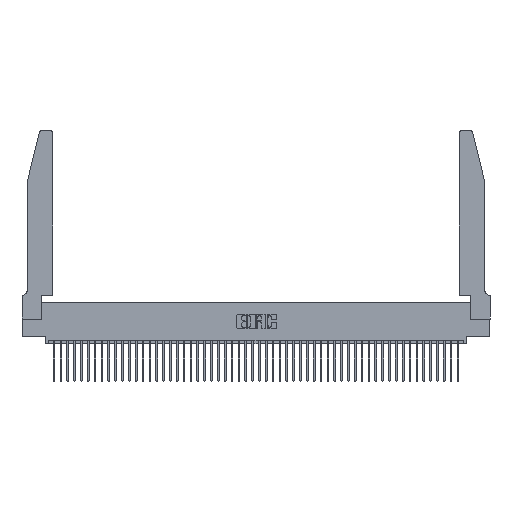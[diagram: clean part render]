
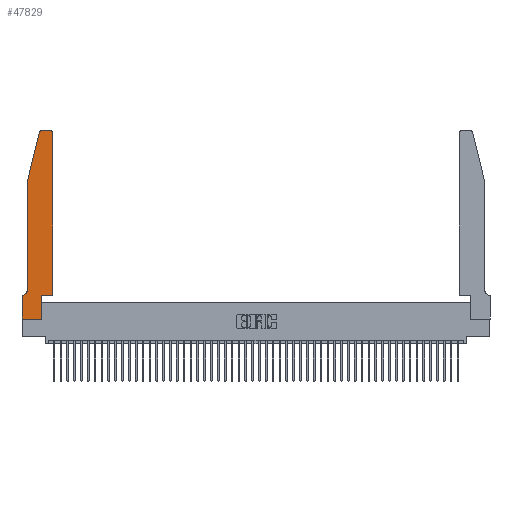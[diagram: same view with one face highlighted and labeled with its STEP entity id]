
A CAD part, top view. The second image highlights one B-rep face of the part: STEP entity #47829.
In plain terms, the highlighted planar face has unit normal (0, 0, 1).
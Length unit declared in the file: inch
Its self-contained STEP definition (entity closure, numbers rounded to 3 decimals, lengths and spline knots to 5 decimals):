
#329 = VERTEX_POINT ( 'NONE', #30062 ) ;
#383 = CARTESIAN_POINT ( 'NONE',  ( 0.2605, 2.75, 0.37 ) ) ;
#395 = LINE ( 'NONE', #383, #38813 ) ;
#433 = DIRECTION ( 'NONE',  ( 0., 0., 1. ) ) ;
#830 = EDGE_CURVE ( 'NONE', #15135, #20562, #17797, .T. ) ;
#2354 = LINE ( 'NONE', #9603, #21689 ) ;
#2930 = CARTESIAN_POINT ( 'NONE',  ( 0., 0., 0.37 ) ) ;
#4308 = DIRECTION ( 'NONE',  ( -1., 0., 0. ) ) ;
#4812 = DIRECTION ( 'NONE',  ( 1., 0., 0. ) ) ;
#5702 = FACE_OUTER_BOUND ( 'NONE', #33697, .T. ) ;
#6238 = CARTESIAN_POINT ( 'NONE',  ( 0.4205, 2.72, 0.37 ) ) ;
#7221 = VECTOR ( 'NONE', #25998, 39.37008 ) ;
#7371 = ORIENTED_EDGE ( 'NONE', *, *, #9291, .T. ) ;
#7664 = CARTESIAN_POINT ( 'NONE',  ( 0.0055, 0.42, 0.37 ) ) ;
#7694 = LINE ( 'NONE', #33181, #29290 ) ;
#8608 = EDGE_CURVE ( 'NONE', #26671, #40325, #7694, .T. ) ;
#9291 = EDGE_CURVE ( 'NONE', #26910, #37167, #21571, .T. ) ;
#9395 = AXIS2_PLACEMENT_3D ( 'NONE', #23550, #433, #27371 ) ;
#9603 = CARTESIAN_POINT ( 'NONE',  ( 0.0755, 2., 0.37 ) ) ;
#10123 = DIRECTION ( 'NONE',  ( 1., 0., 0. ) ) ;
#10576 = VECTOR ( 'NONE', #10858, 39.37008 ) ;
#10702 = CARTESIAN_POINT ( 'NONE',  ( 0.4205, 2.75, 0.37 ) ) ;
#10858 = DIRECTION ( 'NONE',  ( 0., -1., 0. ) ) ;
#11010 = VECTOR ( 'NONE', #29513, 39.37008 ) ;
#11382 = AXIS2_PLACEMENT_3D ( 'NONE', #7664, #34419, #11530 ) ;
#11530 = DIRECTION ( 'NONE',  ( -1., 0., 0. ) ) ;
#12657 = CARTESIAN_POINT ( 'NONE',  ( 0., 0.35, 0.37 ) ) ;
#12676 = CARTESIAN_POINT ( 'NONE',  ( 0.2865, 0.35, 0.37 ) ) ;
#13490 = DIRECTION ( 'NONE',  ( -0.239, -0.971, 0. ) ) ;
#13659 = DIRECTION ( 'NONE',  ( 0., -1., 0. ) ) ;
#14196 = ORIENTED_EDGE ( 'NONE', *, *, #830, .T. ) ;
#14727 = CARTESIAN_POINT ( 'NONE',  ( 0.0755, 0.42, 0.37 ) ) ;
#14884 = CIRCLE ( 'NONE', #9395, 0.03 ) ;
#15135 = VERTEX_POINT ( 'NONE', #15682 ) ;
#15682 = CARTESIAN_POINT ( 'NONE',  ( 0., 0.35, 0.37 ) ) ;
#16291 = CARTESIAN_POINT ( 'NONE',  ( 0.4505, 0.35, 0.37 ) ) ;
#16517 = DIRECTION ( 'NONE',  ( 0., 0., 1. ) ) ;
#17474 = LINE ( 'NONE', #2930, #7221 ) ;
#17797 = LINE ( 'NONE', #21390, #26744 ) ;
#18210 = VECTOR ( 'NONE', #36298, 39.37008 ) ;
#18536 = VERTEX_POINT ( 'NONE', #12676 ) ;
#20562 = VERTEX_POINT ( 'NONE', #30618 ) ;
#20833 = LINE ( 'NONE', #37596, #10576 ) ;
#21390 = CARTESIAN_POINT ( 'NONE',  ( 0., 0., 0.37 ) ) ;
#21571 = CIRCLE ( 'NONE', #11382, 0.07 ) ;
#21681 = ORIENTED_EDGE ( 'NONE', *, *, #34355, .T. ) ;
#21689 = VECTOR ( 'NONE', #13490, 39.37008 ) ;
#23550 = CARTESIAN_POINT ( 'NONE',  ( 0.284, 2.72, 0.37 ) ) ;
#23723 = ORIENTED_EDGE ( 'NONE', *, *, #31315, .T. ) ;
#25989 = ORIENTED_EDGE ( 'NONE', *, *, #30127, .T. ) ;
#25998 = DIRECTION ( 'NONE',  ( 1., 0., 0. ) ) ;
#26346 = EDGE_CURVE ( 'NONE', #20562, #38837, #17474, .T. ) ;
#26671 = VERTEX_POINT ( 'NONE', #46762 ) ;
#26744 = VECTOR ( 'NONE', #13659, 39.37008 ) ;
#26819 = LINE ( 'NONE', #16291, #34550 ) ;
#26881 = VERTEX_POINT ( 'NONE', #10702 ) ;
#26910 = VERTEX_POINT ( 'NONE', #14727 ) ;
#26913 = EDGE_CURVE ( 'NONE', #329, #26910, #20833, .T. ) ;
#26965 = CIRCLE ( 'NONE', #45548, 0.03 ) ;
#27214 = ORIENTED_EDGE ( 'NONE', *, *, #43322, .T. ) ;
#27371 = DIRECTION ( 'NONE',  ( 1., 0., 0. ) ) ;
#28534 = EDGE_CURVE ( 'NONE', #37167, #15135, #31357, .T. ) ;
#29290 = VECTOR ( 'NONE', #36991, 39.37008 ) ;
#29513 = DIRECTION ( 'NONE',  ( -1., 0., 0. ) ) ;
#30062 = CARTESIAN_POINT ( 'NONE',  ( 0.0755, 2., 0.37 ) ) ;
#30127 = EDGE_CURVE ( 'NONE', #32464, #329, #2354, .T. ) ;
#30618 = CARTESIAN_POINT ( 'NONE',  ( 0., 0., 0.37 ) ) ;
#31315 = EDGE_CURVE ( 'NONE', #26881, #47466, #395, .T. ) ;
#31357 = LINE ( 'NONE', #48469, #11010 ) ;
#32105 = ORIENTED_EDGE ( 'NONE', *, *, #36471, .T. ) ;
#32464 = VERTEX_POINT ( 'NONE', #48519 ) ;
#32500 = CARTESIAN_POINT ( 'NONE',  ( 0.2865, 0.35, 0.37 ) ) ;
#32634 = EDGE_CURVE ( 'NONE', #47466, #32464, #14884, .T. ) ;
#33056 = DIRECTION ( 'NONE',  ( 0., 0., 1. ) ) ;
#33181 = CARTESIAN_POINT ( 'NONE',  ( 0.4505, 0.35, 0.37 ) ) ;
#33697 = EDGE_LOOP ( 'NONE', ( #23723, #38238, #25989, #45006, #7371, #46079, #14196, #42785, #32105, #21681, #48264, #27214 ) ) ;
#34355 = EDGE_CURVE ( 'NONE', #18536, #26671, #26819, .T. ) ;
#34419 = DIRECTION ( 'NONE',  ( 0., 0., -1. ) ) ;
#34550 = VECTOR ( 'NONE', #4812, 39.37008 ) ;
#36298 = DIRECTION ( 'NONE',  ( 0., 1., 0. ) ) ;
#36471 = EDGE_CURVE ( 'NONE', #38837, #18536, #38470, .T. ) ;
#36991 = DIRECTION ( 'NONE',  ( 0., 1., 0. ) ) ;
#37167 = VERTEX_POINT ( 'NONE', #48381 ) ;
#37596 = CARTESIAN_POINT ( 'NONE',  ( 0.0755, 2., 0.37 ) ) ;
#38229 = CARTESIAN_POINT ( 'NONE',  ( 0.2865, 0., 0.37 ) ) ;
#38238 = ORIENTED_EDGE ( 'NONE', *, *, #32634, .T. ) ;
#38470 = LINE ( 'NONE', #32500, #18210 ) ;
#38813 = VECTOR ( 'NONE', #4308, 39.37008 ) ;
#38837 = VERTEX_POINT ( 'NONE', #38229 ) ;
#39368 = PLANE ( 'NONE',  #43437 ) ;
#40325 = VERTEX_POINT ( 'NONE', #41491 ) ;
#41491 = CARTESIAN_POINT ( 'NONE',  ( 0.4505, 2.72, 0.37 ) ) ;
#42785 = ORIENTED_EDGE ( 'NONE', *, *, #26346, .T. ) ;
#43184 = DIRECTION ( 'NONE',  ( 1., 0., 0. ) ) ;
#43322 = EDGE_CURVE ( 'NONE', #40325, #26881, #26965, .T. ) ;
#43437 = AXIS2_PLACEMENT_3D ( 'NONE', #12657, #16517, #43184 ) ;
#44896 = CARTESIAN_POINT ( 'NONE',  ( 0.284, 2.75, 0.37 ) ) ;
#45006 = ORIENTED_EDGE ( 'NONE', *, *, #26913, .T. ) ;
#45548 = AXIS2_PLACEMENT_3D ( 'NONE', #6238, #33056, #10123 ) ;
#46079 = ORIENTED_EDGE ( 'NONE', *, *, #28534, .T. ) ;
#46762 = CARTESIAN_POINT ( 'NONE',  ( 0.4505, 0.35, 0.37 ) ) ;
#47466 = VERTEX_POINT ( 'NONE', #44896 ) ;
#47829 = ADVANCED_FACE ( 'NONE', ( #5702 ), #39368, .T. ) ;
#48264 = ORIENTED_EDGE ( 'NONE', *, *, #8608, .T. ) ;
#48381 = CARTESIAN_POINT ( 'NONE',  ( 0.0055, 0.35, 0.37 ) ) ;
#48469 = CARTESIAN_POINT ( 'NONE',  ( 0.0755, 0.35, 0.37 ) ) ;
#48519 = CARTESIAN_POINT ( 'NONE',  ( 0.25487, 2.72718, 0.37 ) ) ;
